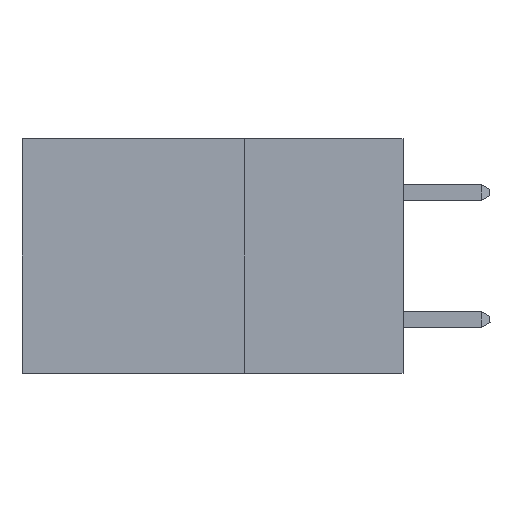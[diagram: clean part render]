
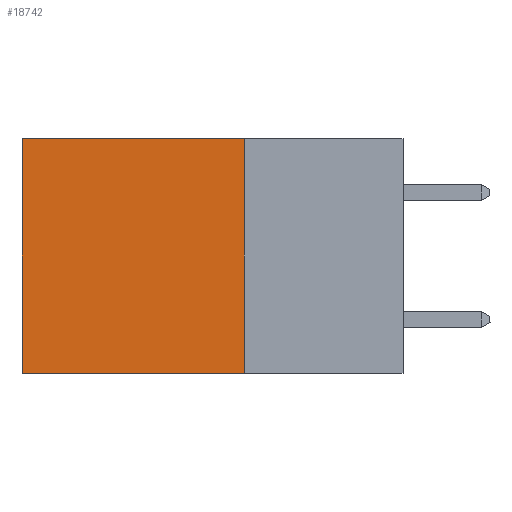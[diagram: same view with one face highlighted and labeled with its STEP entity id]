
A CAD part, left-side view. The second image highlights one B-rep face of the part: STEP entity #18742.
In plain terms, the highlighted planar face has unit normal (-1, 0, 0).
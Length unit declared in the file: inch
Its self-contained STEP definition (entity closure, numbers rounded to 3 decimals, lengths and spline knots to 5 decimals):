
#222 = CARTESIAN_POINT ( 'NONE',  ( 0.2875, 0.6, -0.37 ) ) ;
#979 = VECTOR ( 'NONE', #16107, 39.37008 ) ;
#1887 = CARTESIAN_POINT ( 'NONE',  ( 0.2875, 0.25, -0.37 ) ) ;
#3051 = ORIENTED_EDGE ( 'NONE', *, *, #16637, .F. ) ;
#4855 = CARTESIAN_POINT ( 'NONE',  ( 0.2875, 0.25, -0.37 ) ) ;
#5011 = DIRECTION ( 'NONE',  ( 0., 1., 0. ) ) ;
#6013 = CARTESIAN_POINT ( 'NONE',  ( 0.2875, 0.25, 0. ) ) ;
#6972 = CARTESIAN_POINT ( 'NONE',  ( 0.2875, 0.6, 0. ) ) ;
#8340 = ORIENTED_EDGE ( 'NONE', *, *, #13584, .T. ) ;
#8353 = VECTOR ( 'NONE', #5011, 39.37008 ) ;
#8721 = PLANE ( 'NONE',  #10054 ) ;
#9289 = DIRECTION ( 'NONE',  ( 0., 0., -1. ) ) ;
#9419 = CARTESIAN_POINT ( 'NONE',  ( 0.2875, 0.25, 0. ) ) ;
#9621 = CARTESIAN_POINT ( 'NONE',  ( 0.2875, 0.25, 0. ) ) ;
#10054 = AXIS2_PLACEMENT_3D ( 'NONE', #16039, #11496, #18953 ) ;
#10826 = VERTEX_POINT ( 'NONE', #1887 ) ;
#11496 = DIRECTION ( 'NONE',  ( 1., 0., 0. ) ) ;
#13085 = CARTESIAN_POINT ( 'NONE',  ( 0.2875, 0.6, 0. ) ) ;
#13584 = EDGE_CURVE ( 'NONE', #16542, #19528, #28773, .T. ) ;
#14507 = LINE ( 'NONE', #9621, #14575 ) ;
#14575 = VECTOR ( 'NONE', #9289, 39.37008 ) ;
#14631 = LINE ( 'NONE', #4855, #8353 ) ;
#15849 = EDGE_LOOP ( 'NONE', ( #21034, #3051, #19264, #8340 ) ) ;
#15872 = EDGE_CURVE ( 'NONE', #19528, #25014, #18266, .T. ) ;
#16039 = CARTESIAN_POINT ( 'NONE',  ( 0.2875, 0.25, 0. ) ) ;
#16107 = DIRECTION ( 'NONE',  ( 0., 1., 0. ) ) ;
#16542 = VERTEX_POINT ( 'NONE', #9419 ) ;
#16637 = EDGE_CURVE ( 'NONE', #10826, #25014, #14631, .T. ) ;
#18266 = LINE ( 'NONE', #13085, #21302 ) ;
#18742 = ADVANCED_FACE ( 'NONE', ( #25957 ), #8721, .F. ) ;
#18953 = DIRECTION ( 'NONE',  ( 0., 0., -1. ) ) ;
#19264 = ORIENTED_EDGE ( 'NONE', *, *, #31828, .F. ) ;
#19528 = VERTEX_POINT ( 'NONE', #6972 ) ;
#21034 = ORIENTED_EDGE ( 'NONE', *, *, #15872, .T. ) ;
#21302 = VECTOR ( 'NONE', #30452, 39.37008 ) ;
#25014 = VERTEX_POINT ( 'NONE', #222 ) ;
#25957 = FACE_OUTER_BOUND ( 'NONE', #15849, .T. ) ;
#28773 = LINE ( 'NONE', #6013, #979 ) ;
#30452 = DIRECTION ( 'NONE',  ( 0., 0., -1. ) ) ;
#31828 = EDGE_CURVE ( 'NONE', #16542, #10826, #14507, .T. ) ;
